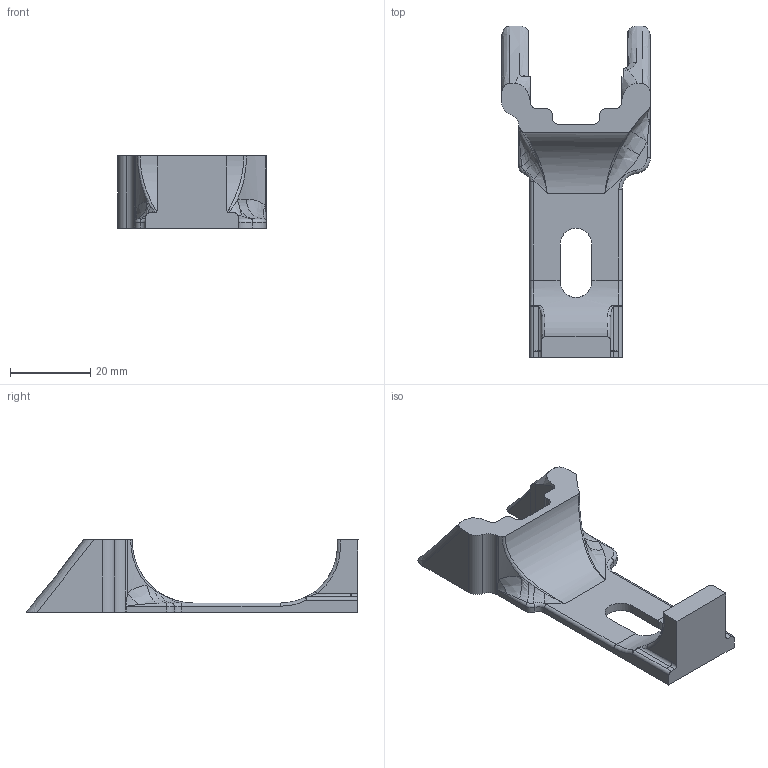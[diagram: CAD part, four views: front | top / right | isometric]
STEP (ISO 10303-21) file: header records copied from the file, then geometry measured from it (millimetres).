
FILE_DESCRIPTION (( 'STEP AP214' ), '1' );
FILE_NAME ('3.STEP', '2013-09-29T07:12:14', ( 'elpi' ), ( '' ), 'SwSTEP 2.0', 'SolidWorks 2013', '' );
FILE_SCHEMA (( 'AUTOMOTIVE_DESIGN' ));
Length unit declared in the file: millimetre
Products named in the file (1): 3
Bounding box: 37.13 x 82.97 x 18.09 mm (x, y, z)
Volume: 12177.7 mm3; surface area: 6535.3 mm2
Topology: 1 solids, 1 shells, 113 faces, 301 edges, 185 vertices
Faces by surface type: cylinder 35, bspline 33, plane 32, torus 12, sphere 1
Entity records: 5372 total; most frequent: CARTESIAN_POINT 2795, ORIENTED_EDGE 594, DIRECTION 453, EDGE_CURVE 297, VERTEX_POINT 185, AXIS2_PLACEMENT_3D 167, VECTOR 119, LINE 119
